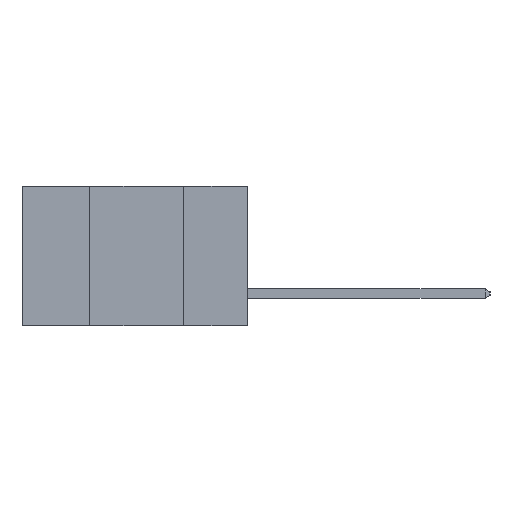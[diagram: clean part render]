
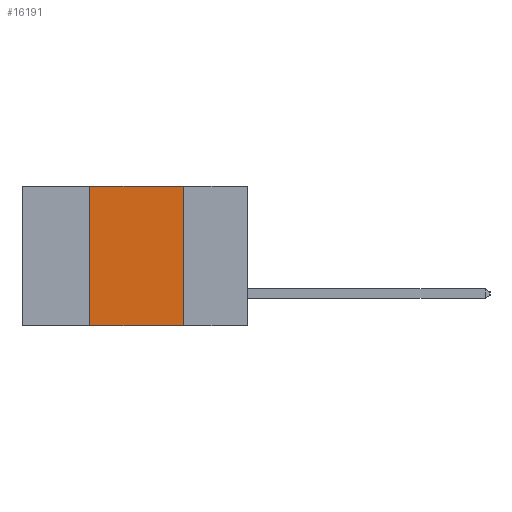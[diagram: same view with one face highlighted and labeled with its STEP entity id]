
A CAD part, left-side view. The second image highlights one B-rep face of the part: STEP entity #16191.
In plain terms, the highlighted planar face has unit normal (-1, 0, 0).
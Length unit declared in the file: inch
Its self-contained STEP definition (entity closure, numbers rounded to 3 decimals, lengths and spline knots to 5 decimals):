
#608 = CARTESIAN_POINT ( 'NONE',  ( 0., 0.6, 0. ) ) ;
#616 = VECTOR ( 'NONE', #18119, 39.37008 ) ;
#937 = VERTEX_POINT ( 'NONE', #9936 ) ;
#1536 = CARTESIAN_POINT ( 'NONE',  ( 0., 0.6, -0.37 ) ) ;
#2099 = PLANE ( 'NONE',  #4755 ) ;
#2171 = ORIENTED_EDGE ( 'NONE', *, *, #12876, .T. ) ;
#2248 = LINE ( 'NONE', #8155, #17141 ) ;
#2255 = VERTEX_POINT ( 'NONE', #8887 ) ;
#2325 = VERTEX_POINT ( 'NONE', #3152 ) ;
#3023 = DIRECTION ( 'NONE',  ( 0., -1., 0. ) ) ;
#3152 = CARTESIAN_POINT ( 'NONE',  ( 0., 0.42, 0. ) ) ;
#3618 = DIRECTION ( 'NONE',  ( 0., 0., -1. ) ) ;
#4572 = LINE ( 'NONE', #14036, #616 ) ;
#4755 = AXIS2_PLACEMENT_3D ( 'NONE', #608, #12364, #3618 ) ;
#5060 = EDGE_CURVE ( 'NONE', #937, #2325, #2248, .T. ) ;
#6266 = CARTESIAN_POINT ( 'NONE',  ( 0., 0.17, -0.37 ) ) ;
#6618 = ORIENTED_EDGE ( 'NONE', *, *, #16949, .F. ) ;
#7535 = ORIENTED_EDGE ( 'NONE', *, *, #13240, .F. ) ;
#7626 = FACE_OUTER_BOUND ( 'NONE', #11442, .T. ) ;
#8044 = DIRECTION ( 'NONE',  ( 0., 0., 1. ) ) ;
#8155 = CARTESIAN_POINT ( 'NONE',  ( 0., 0.42, -0.37 ) ) ;
#8211 = DIRECTION ( 'NONE',  ( 0., 0., -1. ) ) ;
#8537 = VERTEX_POINT ( 'NONE', #6266 ) ;
#8556 = VECTOR ( 'NONE', #8211, 39.37008 ) ;
#8887 = CARTESIAN_POINT ( 'NONE',  ( 0., 0.17, 0. ) ) ;
#9936 = CARTESIAN_POINT ( 'NONE',  ( 0., 0.42, -0.37 ) ) ;
#11056 = LINE ( 'NONE', #1536, #17995 ) ;
#11442 = EDGE_LOOP ( 'NONE', ( #7535, #6618, #17885, #2171 ) ) ;
#12364 = DIRECTION ( 'NONE',  ( 1., 0., 0. ) ) ;
#12384 = LINE ( 'NONE', #18036, #8556 ) ;
#12876 = EDGE_CURVE ( 'NONE', #937, #8537, #11056, .T. ) ;
#13240 = EDGE_CURVE ( 'NONE', #2255, #8537, #12384, .T. ) ;
#14036 = CARTESIAN_POINT ( 'NONE',  ( 0., 0.6, 0. ) ) ;
#16191 = ADVANCED_FACE ( 'NONE', ( #7626 ), #2099, .F. ) ;
#16949 = EDGE_CURVE ( 'NONE', #2325, #2255, #4572, .T. ) ;
#17141 = VECTOR ( 'NONE', #8044, 39.37008 ) ;
#17885 = ORIENTED_EDGE ( 'NONE', *, *, #5060, .F. ) ;
#17995 = VECTOR ( 'NONE', #3023, 39.37008 ) ;
#18036 = CARTESIAN_POINT ( 'NONE',  ( 0., 0.17, -0.37 ) ) ;
#18119 = DIRECTION ( 'NONE',  ( 0., -1., 0. ) ) ;
